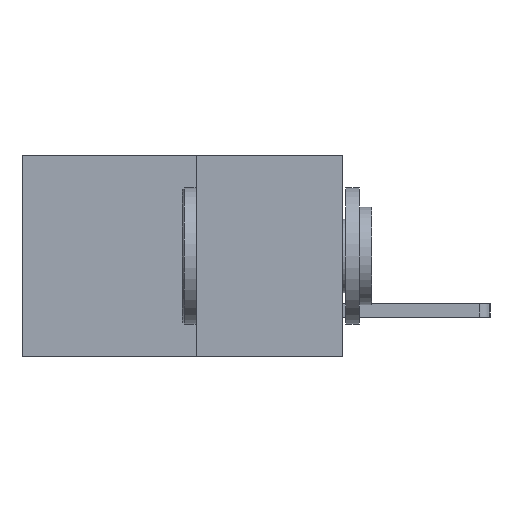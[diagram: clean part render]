
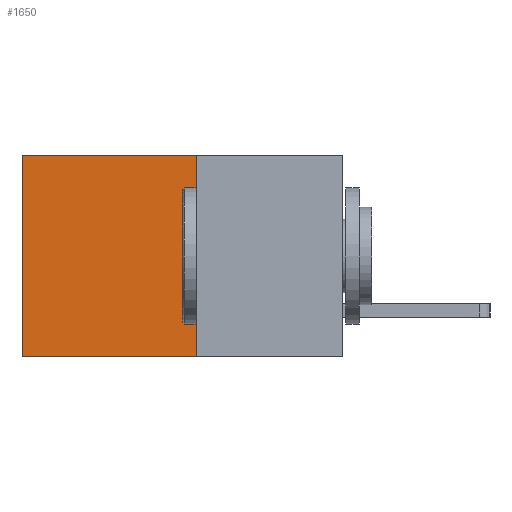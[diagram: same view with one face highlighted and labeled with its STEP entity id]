
A CAD part, left-side view. The second image highlights one B-rep face of the part: STEP entity #1650.
In plain terms, the highlighted planar face has unit normal (-1, 0, 0).
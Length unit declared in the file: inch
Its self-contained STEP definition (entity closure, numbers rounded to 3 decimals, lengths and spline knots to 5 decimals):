
#482 = VECTOR ( 'NONE', #1572, 39.37008 ) ;
#707 = DIRECTION ( 'NONE',  ( 0., 1., 0. ) ) ;
#880 = EDGE_CURVE ( 'NONE', #2023, #1482, #2594, .T. ) ;
#1482 = VERTEX_POINT ( 'NONE', #7188 ) ;
#1572 = DIRECTION ( 'NONE',  ( 0., 1., 0. ) ) ;
#1645 = CARTESIAN_POINT ( 'NONE',  ( 0.277, 0.27, -0.37 ) ) ;
#1650 = ADVANCED_FACE ( 'NONE', ( #5942 ), #5802, .F. ) ;
#1904 = VECTOR ( 'NONE', #7197, 39.37008 ) ;
#2023 = VERTEX_POINT ( 'NONE', #9566 ) ;
#2588 = CARTESIAN_POINT ( 'NONE',  ( 0.277, 0.27, 0. ) ) ;
#2594 = LINE ( 'NONE', #2588, #482 ) ;
#3062 = CARTESIAN_POINT ( 'NONE',  ( 0.277, 0.27, -0.37 ) ) ;
#3203 = DIRECTION ( 'NONE',  ( 0., 0., -1. ) ) ;
#3588 = LINE ( 'NONE', #3062, #7557 ) ;
#4186 = ORIENTED_EDGE ( 'NONE', *, *, #9855, .F. ) ;
#4875 = EDGE_LOOP ( 'NONE', ( #9617, #4186, #9834, #9755 ) ) ;
#5615 = CARTESIAN_POINT ( 'NONE',  ( 0.277, 0.59, -0.37 ) ) ;
#5802 = PLANE ( 'NONE',  #10182 ) ;
#5942 = FACE_OUTER_BOUND ( 'NONE', #4875, .T. ) ;
#6297 = CARTESIAN_POINT ( 'NONE',  ( 0.277, 0.59, -0.37 ) ) ;
#6353 = DIRECTION ( 'NONE',  ( 0., 0., -1. ) ) ;
#6371 = DIRECTION ( 'NONE',  ( 1., 0., 0. ) ) ;
#6460 = VECTOR ( 'NONE', #3203, 39.37008 ) ;
#6536 = VERTEX_POINT ( 'NONE', #6297 ) ;
#6718 = LINE ( 'NONE', #5615, #6460 ) ;
#6889 = VERTEX_POINT ( 'NONE', #7645 ) ;
#7188 = CARTESIAN_POINT ( 'NONE',  ( 0.277, 0.59, 0. ) ) ;
#7197 = DIRECTION ( 'NONE',  ( 0., 0., -1. ) ) ;
#7557 = VECTOR ( 'NONE', #707, 39.37008 ) ;
#7645 = CARTESIAN_POINT ( 'NONE',  ( 0.277, 0.27, -0.37 ) ) ;
#8069 = EDGE_CURVE ( 'NONE', #2023, #6889, #8201, .T. ) ;
#8201 = LINE ( 'NONE', #1645, #1904 ) ;
#9308 = EDGE_CURVE ( 'NONE', #1482, #6536, #6718, .T. ) ;
#9380 = CARTESIAN_POINT ( 'NONE',  ( 0.277, 0.27, -0.37 ) ) ;
#9566 = CARTESIAN_POINT ( 'NONE',  ( 0.277, 0.27, 0. ) ) ;
#9617 = ORIENTED_EDGE ( 'NONE', *, *, #9308, .T. ) ;
#9755 = ORIENTED_EDGE ( 'NONE', *, *, #880, .T. ) ;
#9834 = ORIENTED_EDGE ( 'NONE', *, *, #8069, .F. ) ;
#9855 = EDGE_CURVE ( 'NONE', #6889, #6536, #3588, .T. ) ;
#10182 = AXIS2_PLACEMENT_3D ( 'NONE', #9380, #6371, #6353 ) ;
